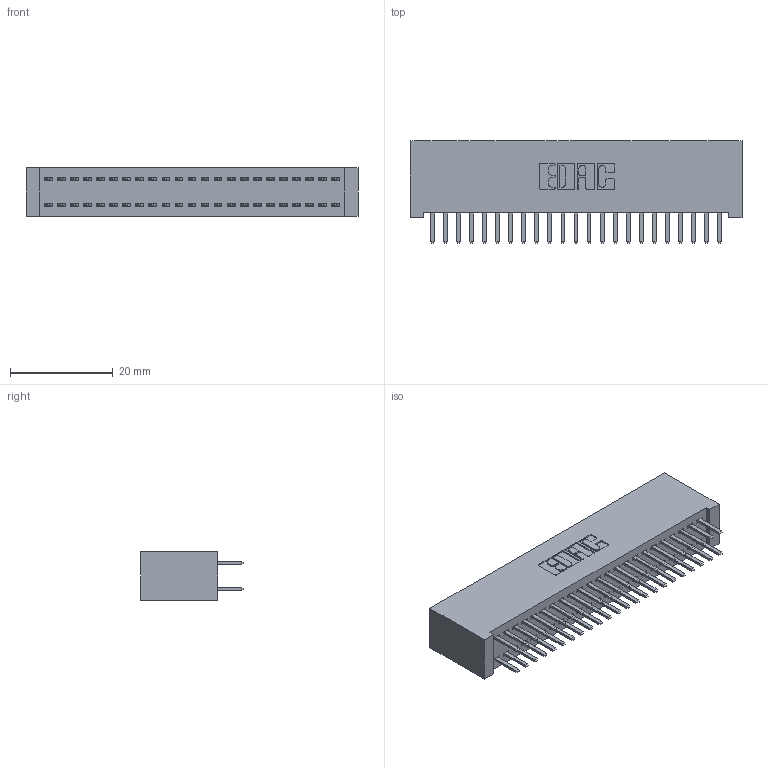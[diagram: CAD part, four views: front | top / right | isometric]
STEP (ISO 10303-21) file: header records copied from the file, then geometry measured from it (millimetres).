
FILE_DESCRIPTION (( 'STEP AP203' ), '1' );
FILE_NAME ('392-046-520-201.STEP', '2019-10-07T23:18:22', ( '' ), ( '' ), 'SwSTEP 2.0', 'SolidWorks 2016', '' );
FILE_SCHEMA (( 'CONFIG_CONTROL_DESIGN' ));
Length unit declared in the file: inch
Products named in the file (3): 345-292-001_345-293-120; 392-046-520-201; 342 Part_Lugless
Assembly tree (47 placements, depth 2):
  392-046-520-201
    342 Part_Lugless
    345-292-001_345-293-120  x46
Bounding box: 64.67 x 20.02 x 9.4 mm (x, y, z)
Volume: 6139.8 mm3; surface area: 9924.4 mm2
Topology: 47 solids, 47 shells, 2678 faces, 7773 edges, 5058 vertices
Faces by surface type: plane 1810, cylinder 868
Entity records: 16959 total; most frequent: CARTESIAN_POINT 2842, ORIENTED_EDGE 2766, DIRECTION 2443, EDGE_CURVE 1383, VECTOR 1259, LINE 1259, VERTEX_POINT 918, AXIS2_PLACEMENT_3D 592
